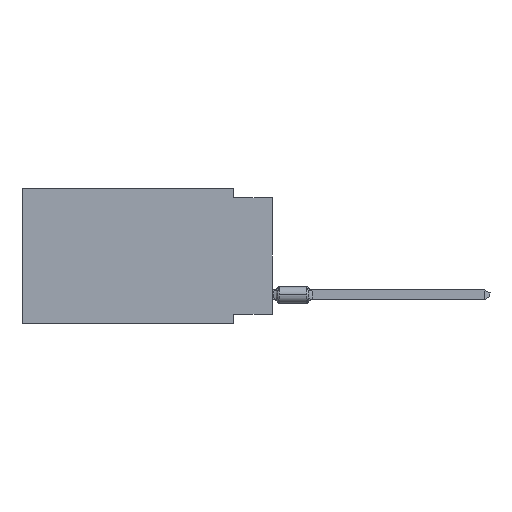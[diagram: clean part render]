
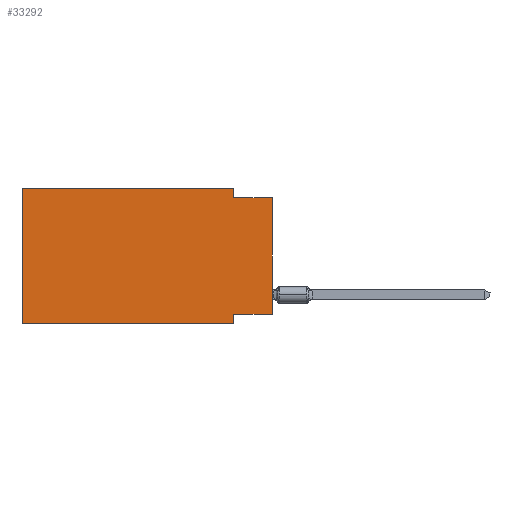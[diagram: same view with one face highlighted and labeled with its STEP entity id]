
A CAD part, left-side view. The second image highlights one B-rep face of the part: STEP entity #33292.
In plain terms, the highlighted planar face has unit normal (-1, 0, 0).
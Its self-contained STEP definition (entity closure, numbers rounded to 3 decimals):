
#3062 = FACE_OUTER_BOUND ( 'NONE', #40256, .T. ) ;
#3871 = ORIENTED_EDGE ( 'NONE', *, *, #21699, .F. ) ;
#5420 = EDGE_CURVE ( 'NONE', #23425, #9755, #45057, .T. ) ;
#6040 = VECTOR ( 'NONE', #48843, 1000. ) ;
#6451 = CARTESIAN_POINT ( 'NONE',  ( 0., 16.383, 0. ) ) ;
#7509 = ORIENTED_EDGE ( 'NONE', *, *, #5420, .F. ) ;
#8420 = DIRECTION ( 'NONE',  ( 0., 0., -1. ) ) ;
#9755 = VERTEX_POINT ( 'NONE', #52181 ) ;
#9787 = AXIS2_PLACEMENT_3D ( 'NONE', #24213, #37433, #24759 ) ;
#10007 = VECTOR ( 'NONE', #27028, 1000. ) ;
#10717 = ORIENTED_EDGE ( 'NONE', *, *, #29133, .T. ) ;
#11436 = VECTOR ( 'NONE', #47058, 1000. ) ;
#12785 = VECTOR ( 'NONE', #44827, 1000. ) ;
#13619 = VERTEX_POINT ( 'NONE', #42679 ) ;
#14073 = EDGE_CURVE ( 'NONE', #28309, #26628, #29863, .T. ) ;
#14350 = CARTESIAN_POINT ( 'NONE',  ( 0., 0., -8.255 ) ) ;
#14732 = ORIENTED_EDGE ( 'NONE', *, *, #26950, .T. ) ;
#15760 = VECTOR ( 'NONE', #17519, 1000. ) ;
#17519 = DIRECTION ( 'NONE',  ( 0., 0., 1. ) ) ;
#17870 = CARTESIAN_POINT ( 'NONE',  ( 0., 0., 0. ) ) ;
#18194 = ORIENTED_EDGE ( 'NONE', *, *, #23950, .F. ) ;
#20256 = PLANE ( 'NONE',  #9787 ) ;
#20261 = CARTESIAN_POINT ( 'NONE',  ( 0., 2.54, 0. ) ) ;
#20994 = CARTESIAN_POINT ( 'NONE',  ( 0., 0., -0.635 ) ) ;
#21394 = ORIENTED_EDGE ( 'NONE', *, *, #14073, .F. ) ;
#21699 = EDGE_CURVE ( 'NONE', #9755, #28309, #25606, .T. ) ;
#22290 = CARTESIAN_POINT ( 'NONE',  ( 0., 16.383, 0. ) ) ;
#22864 = LINE ( 'NONE', #40037, #12785 ) ;
#23425 = VERTEX_POINT ( 'NONE', #25210 ) ;
#23950 = EDGE_CURVE ( 'NONE', #41063, #23425, #42854, .T. ) ;
#24213 = CARTESIAN_POINT ( 'NONE',  ( 0., 16.383, 0. ) ) ;
#24476 = DIRECTION ( 'NONE',  ( 0., -1., 0. ) ) ;
#24759 = DIRECTION ( 'NONE',  ( 0., 0., -1. ) ) ;
#25136 = VECTOR ( 'NONE', #24476, 1000. ) ;
#25210 = CARTESIAN_POINT ( 'NONE',  ( 0., 16.383, 0. ) ) ;
#25606 = LINE ( 'NONE', #20261, #38133 ) ;
#26628 = VERTEX_POINT ( 'NONE', #20994 ) ;
#26950 = EDGE_CURVE ( 'NONE', #37395, #26628, #30531, .T. ) ;
#27028 = DIRECTION ( 'NONE',  ( 0., 1., 0. ) ) ;
#28309 = VERTEX_POINT ( 'NONE', #41409 ) ;
#29133 = EDGE_CURVE ( 'NONE', #41063, #30887, #22864, .T. ) ;
#29549 = EDGE_CURVE ( 'NONE', #37395, #13619, #52665, .T. ) ;
#29863 = LINE ( 'NONE', #43097, #11436 ) ;
#30193 = CARTESIAN_POINT ( 'NONE',  ( 0., 2.54, -8.89 ) ) ;
#30531 = LINE ( 'NONE', #17870, #32287 ) ;
#30887 = VERTEX_POINT ( 'NONE', #30193 ) ;
#32287 = VECTOR ( 'NONE', #43219, 1000. ) ;
#33292 = ADVANCED_FACE ( 'NONE', ( #3062 ), #20256, .F. ) ;
#34941 = ORIENTED_EDGE ( 'NONE', *, *, #49902, .F. ) ;
#35776 = ORIENTED_EDGE ( 'NONE', *, *, #29549, .F. ) ;
#36592 = CARTESIAN_POINT ( 'NONE',  ( 0., 16.383, -8.89 ) ) ;
#37395 = VERTEX_POINT ( 'NONE', #41869 ) ;
#37433 = DIRECTION ( 'NONE',  ( 1., 0., 0. ) ) ;
#38133 = VECTOR ( 'NONE', #8420, 1000. ) ;
#40037 = CARTESIAN_POINT ( 'NONE',  ( 0., 16.383, -8.89 ) ) ;
#40256 = EDGE_LOOP ( 'NONE', ( #14732, #21394, #3871, #7509, #18194, #10717, #34941, #35776 ) ) ;
#41063 = VERTEX_POINT ( 'NONE', #36592 ) ;
#41409 = CARTESIAN_POINT ( 'NONE',  ( 0., 2.54, -0.635 ) ) ;
#41869 = CARTESIAN_POINT ( 'NONE',  ( 0., 0., -8.255 ) ) ;
#42679 = CARTESIAN_POINT ( 'NONE',  ( 0., 2.54, -8.255 ) ) ;
#42854 = LINE ( 'NONE', #22290, #15760 ) ;
#43097 = CARTESIAN_POINT ( 'NONE',  ( 0., 0., -0.635 ) ) ;
#43219 = DIRECTION ( 'NONE',  ( 0., 0., 1. ) ) ;
#44827 = DIRECTION ( 'NONE',  ( 0., -1., 0. ) ) ;
#45057 = LINE ( 'NONE', #6451, #25136 ) ;
#47058 = DIRECTION ( 'NONE',  ( 0., -1., 0. ) ) ;
#48843 = DIRECTION ( 'NONE',  ( 0., 0., -1. ) ) ;
#49396 = CARTESIAN_POINT ( 'NONE',  ( 0., 2.54, -8.89 ) ) ;
#49902 = EDGE_CURVE ( 'NONE', #13619, #30887, #53359, .T. ) ;
#52181 = CARTESIAN_POINT ( 'NONE',  ( 0., 2.54, 0. ) ) ;
#52665 = LINE ( 'NONE', #14350, #10007 ) ;
#53359 = LINE ( 'NONE', #49396, #6040 ) ;
